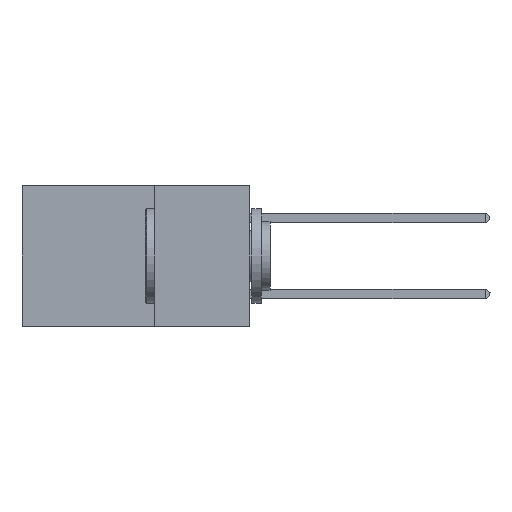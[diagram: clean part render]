
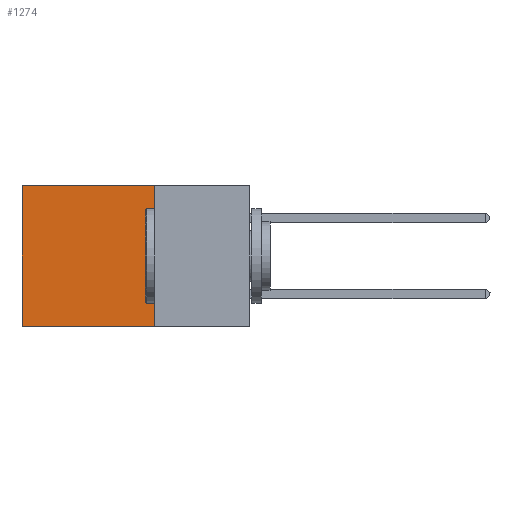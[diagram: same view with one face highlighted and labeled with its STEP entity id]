
A CAD part, left-side view. The second image highlights one B-rep face of the part: STEP entity #1274.
In plain terms, the highlighted planar face has unit normal (-1, 0, 0).
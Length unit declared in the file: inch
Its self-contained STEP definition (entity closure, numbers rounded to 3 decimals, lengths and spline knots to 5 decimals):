
#1274 = ADVANCED_FACE ( 'NONE', ( #23589 ), #28348, .F. ) ;
#2975 = LINE ( 'NONE', #5555, #23725 ) ;
#3180 = ORIENTED_EDGE ( 'NONE', *, *, #4658, .T. ) ;
#3879 = CARTESIAN_POINT ( 'NONE',  ( 0.2875, 0.25, 0. ) ) ;
#4449 = CARTESIAN_POINT ( 'NONE',  ( 0.2875, 0.6, 0. ) ) ;
#4658 = EDGE_CURVE ( 'NONE', #20368, #16380, #10793, .T. ) ;
#5164 = VECTOR ( 'NONE', #27251, 39.37008 ) ;
#5555 = CARTESIAN_POINT ( 'NONE',  ( 0.2875, 0.25, -0.37 ) ) ;
#6525 = VERTEX_POINT ( 'NONE', #13425 ) ;
#8168 = VECTOR ( 'NONE', #9978, 39.37008 ) ;
#9025 = EDGE_LOOP ( 'NONE', ( #3180, #16883, #9940, #9806 ) ) ;
#9806 = ORIENTED_EDGE ( 'NONE', *, *, #19149, .T. ) ;
#9940 = ORIENTED_EDGE ( 'NONE', *, *, #26650, .F. ) ;
#9978 = DIRECTION ( 'NONE',  ( 0., 1., 0. ) ) ;
#9984 = CARTESIAN_POINT ( 'NONE',  ( 0.2875, 0.25, 0. ) ) ;
#10262 = CARTESIAN_POINT ( 'NONE',  ( 0.2875, 0.25, 0. ) ) ;
#10661 = DIRECTION ( 'NONE',  ( 0., 0., -1. ) ) ;
#10793 = LINE ( 'NONE', #4449, #5164 ) ;
#12547 = CARTESIAN_POINT ( 'NONE',  ( 0.2875, 0.25, 0. ) ) ;
#13425 = CARTESIAN_POINT ( 'NONE',  ( 0.2875, 0.25, -0.37 ) ) ;
#13744 = CARTESIAN_POINT ( 'NONE',  ( 0.2875, 0.6, -0.37 ) ) ;
#14174 = LINE ( 'NONE', #12547, #8168 ) ;
#15178 = DIRECTION ( 'NONE',  ( 0., 0., -1. ) ) ;
#16380 = VERTEX_POINT ( 'NONE', #13744 ) ;
#16883 = ORIENTED_EDGE ( 'NONE', *, *, #28950, .F. ) ;
#19149 = EDGE_CURVE ( 'NONE', #29030, #20368, #14174, .T. ) ;
#19417 = VECTOR ( 'NONE', #10661, 39.37008 ) ;
#20368 = VERTEX_POINT ( 'NONE', #22757 ) ;
#21868 = LINE ( 'NONE', #3879, #19417 ) ;
#22757 = CARTESIAN_POINT ( 'NONE',  ( 0.2875, 0.6, 0. ) ) ;
#23589 = FACE_OUTER_BOUND ( 'NONE', #9025, .T. ) ;
#23725 = VECTOR ( 'NONE', #25885, 39.37008 ) ;
#23821 = DIRECTION ( 'NONE',  ( 1., 0., 0. ) ) ;
#25885 = DIRECTION ( 'NONE',  ( 0., 1., 0. ) ) ;
#26650 = EDGE_CURVE ( 'NONE', #29030, #6525, #21868, .T. ) ;
#27251 = DIRECTION ( 'NONE',  ( 0., 0., -1. ) ) ;
#28348 = PLANE ( 'NONE',  #28849 ) ;
#28849 = AXIS2_PLACEMENT_3D ( 'NONE', #10262, #23821, #15178 ) ;
#28950 = EDGE_CURVE ( 'NONE', #6525, #16380, #2975, .T. ) ;
#29030 = VERTEX_POINT ( 'NONE', #9984 ) ;
